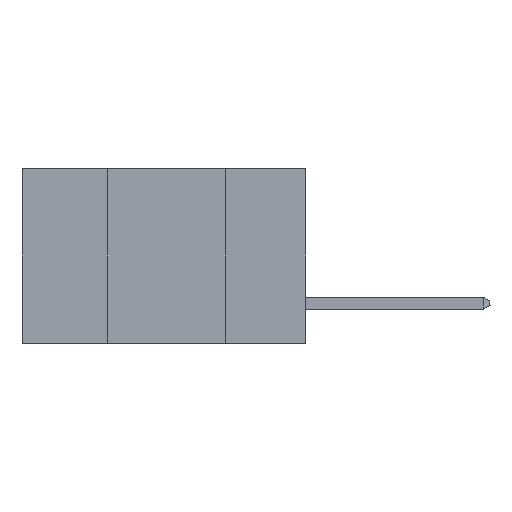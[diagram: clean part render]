
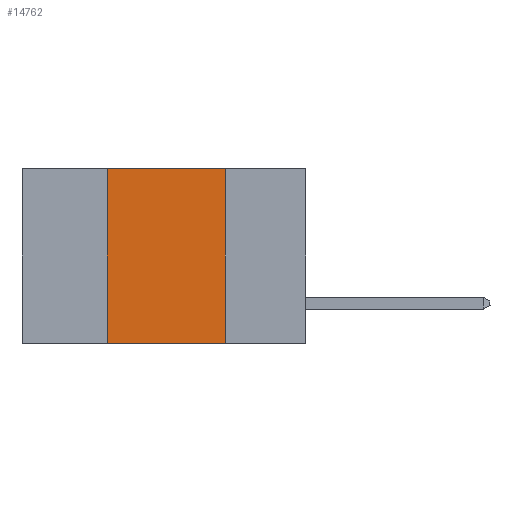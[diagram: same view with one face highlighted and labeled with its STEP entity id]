
A CAD part, left-side view. The second image highlights one B-rep face of the part: STEP entity #14762.
In plain terms, the highlighted planar face has unit normal (-1, 0, 0).
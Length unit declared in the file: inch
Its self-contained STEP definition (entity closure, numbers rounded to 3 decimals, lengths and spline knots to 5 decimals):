
#285 = VECTOR ( 'NONE', #18236, 39.37008 ) ;
#1266 = VERTEX_POINT ( 'NONE', #17552 ) ;
#2058 = VECTOR ( 'NONE', #16631, 39.37008 ) ;
#2997 = FACE_OUTER_BOUND ( 'NONE', #20419, .T. ) ;
#3333 = CARTESIAN_POINT ( 'NONE',  ( 0., 0.17, -0.37 ) ) ;
#4243 = CARTESIAN_POINT ( 'NONE',  ( 0., 0.42, 0. ) ) ;
#4480 = AXIS2_PLACEMENT_3D ( 'NONE', #14410, #5719, #11107 ) ;
#4589 = VERTEX_POINT ( 'NONE', #3333 ) ;
#5719 = DIRECTION ( 'NONE',  ( 1., 0., 0. ) ) ;
#5994 = DIRECTION ( 'NONE',  ( 0., 0., 1. ) ) ;
#6240 = CARTESIAN_POINT ( 'NONE',  ( 0., 0.6, -0.37 ) ) ;
#7897 = LINE ( 'NONE', #6240, #12487 ) ;
#8045 = EDGE_CURVE ( 'NONE', #1266, #21924, #12547, .T. ) ;
#8983 = CARTESIAN_POINT ( 'NONE',  ( 0., 0.17, 0. ) ) ;
#9344 = ORIENTED_EDGE ( 'NONE', *, *, #8045, .F. ) ;
#10582 = LINE ( 'NONE', #4243, #21306 ) ;
#11107 = DIRECTION ( 'NONE',  ( 0., 0., -1. ) ) ;
#11305 = CARTESIAN_POINT ( 'NONE',  ( 0., 0.17, 0. ) ) ;
#12352 = ORIENTED_EDGE ( 'NONE', *, *, #13127, .F. ) ;
#12487 = VECTOR ( 'NONE', #18114, 39.37008 ) ;
#12547 = LINE ( 'NONE', #18487, #2058 ) ;
#13127 = EDGE_CURVE ( 'NONE', #21924, #4589, #21406, .T. ) ;
#14410 = CARTESIAN_POINT ( 'NONE',  ( 0., 0.6, 0. ) ) ;
#14762 = ADVANCED_FACE ( 'NONE', ( #2997 ), #21360, .F. ) ;
#15420 = VERTEX_POINT ( 'NONE', #18684 ) ;
#15988 = ORIENTED_EDGE ( 'NONE', *, *, #21435, .T. ) ;
#16631 = DIRECTION ( 'NONE',  ( 0., -1., 0. ) ) ;
#17552 = CARTESIAN_POINT ( 'NONE',  ( 0., 0.42, 0. ) ) ;
#18114 = DIRECTION ( 'NONE',  ( 0., -1., 0. ) ) ;
#18134 = EDGE_CURVE ( 'NONE', #15420, #1266, #10582, .T. ) ;
#18236 = DIRECTION ( 'NONE',  ( 0., 0., -1. ) ) ;
#18487 = CARTESIAN_POINT ( 'NONE',  ( 0., 0.6, 0. ) ) ;
#18684 = CARTESIAN_POINT ( 'NONE',  ( 0., 0.42, -0.37 ) ) ;
#20419 = EDGE_LOOP ( 'NONE', ( #12352, #9344, #20527, #15988 ) ) ;
#20527 = ORIENTED_EDGE ( 'NONE', *, *, #18134, .F. ) ;
#21306 = VECTOR ( 'NONE', #5994, 39.37008 ) ;
#21360 = PLANE ( 'NONE',  #4480 ) ;
#21406 = LINE ( 'NONE', #11305, #285 ) ;
#21435 = EDGE_CURVE ( 'NONE', #15420, #4589, #7897, .T. ) ;
#21924 = VERTEX_POINT ( 'NONE', #8983 ) ;
